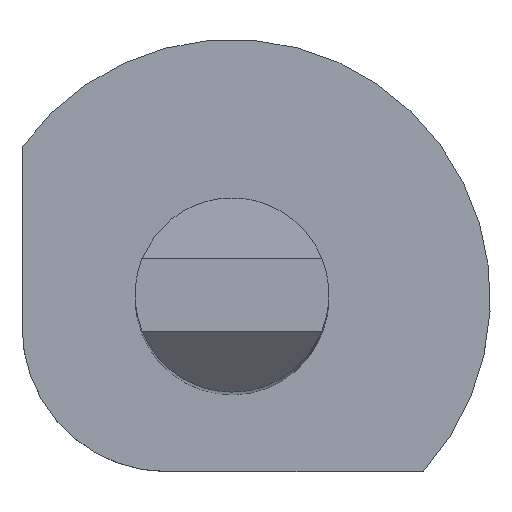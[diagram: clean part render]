
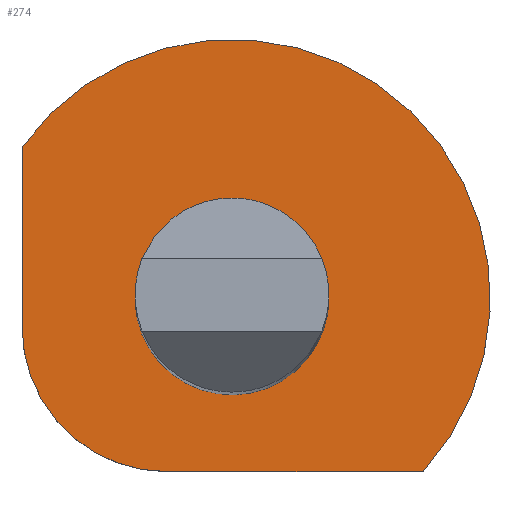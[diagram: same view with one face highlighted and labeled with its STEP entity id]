
A CAD part, top view. The second image highlights one B-rep face of the part: STEP entity #274.
In plain terms, the highlighted planar face has unit normal (0, 0, 1).
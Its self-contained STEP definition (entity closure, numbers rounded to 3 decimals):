
#157=CARTESIAN_POINT('',(2.641,-2.4,0.0));
#158=VERTEX_POINT('',#157);
#165=CARTESIAN_POINT('',(-0.9,-2.4,0.0));
#166=VERTEX_POINT('',#165);
#167=CARTESIAN_POINT('',(2.641,-2.4,0.0));
#168=DIRECTION('',(-1.0,0.0,0.0));
#169=VECTOR('',#168,3.541);
#170=LINE('',#167,#169);
#171=EDGE_CURVE('',#158,#166,#170,.T.);
#197=CARTESIAN_POINT('',(-2.9,-0.4,0.0));
#198=VERTEX_POINT('',#197);
#199=CARTESIAN_POINT('',(-0.9,-0.4,0.0));
#200=DIRECTION('',(0.0,0.0,-1.0));
#201=DIRECTION('',(1.0,0.0,0.0));
#202=AXIS2_PLACEMENT_3D('',#199,#200,#201);
#203=CIRCLE('',#202,2.0);
#204=EDGE_CURVE('',#166,#198,#203,.T.);
#229=CARTESIAN_POINT('',(-2.9,2.08,0.0));
#230=VERTEX_POINT('',#229);
#231=CARTESIAN_POINT('',(-2.9,-0.4,0.0));
#232=DIRECTION('',(0.0,1.0,0.0));
#233=VECTOR('',#232,2.48);
#234=LINE('',#231,#233);
#235=EDGE_CURVE('',#198,#230,#234,.T.);
#246=CARTESIAN_POINT('',(0.0,0.0,0.0));
#247=DIRECTION('',(0.0,0.0,-1.0));
#248=DIRECTION('',(-1.0,0.0,0.0));
#249=AXIS2_PLACEMENT_3D('',#246,#247,#248);
#250=PLANE('',#249);
#251=ORIENTED_EDGE('',*,*,#235,.F.);
#252=ORIENTED_EDGE('',*,*,#204,.F.);
#253=ORIENTED_EDGE('',*,*,#171,.F.);
#254=CARTESIAN_POINT('',(0.0,0.0,0.0));
#255=DIRECTION('',(0.0,0.0,-1.0));
#256=DIRECTION('',(-1.0,0.0,0.0));
#257=AXIS2_PLACEMENT_3D('',#254,#255,#256);
#258=CIRCLE('',#257,3.569);
#259=EDGE_CURVE('',#230,#158,#258,.T.);
#260=ORIENTED_EDGE('',*,*,#259,.F.);
#261=EDGE_LOOP('',(#251,#252,#253,#260));
#262=FACE_OUTER_BOUND('',#261,.T.);
#263=CARTESIAN_POINT('',(1.34,0.,0.0));
#264=VERTEX_POINT('',#263);
#265=CARTESIAN_POINT('',(0.0,0.0,0.0));
#266=DIRECTION('',(0.0,0.0,-1.0));
#267=DIRECTION('',(-1.0,0.0,0.0));
#268=AXIS2_PLACEMENT_3D('',#265,#266,#267);
#269=CIRCLE('',#268,1.34);
#270=EDGE_CURVE('',#264,#264,#269,.T.);
#271=ORIENTED_EDGE('',*,*,#270,.T.);
#272=EDGE_LOOP('',(#271));
#273=FACE_BOUND('',#272,.T.);
#274=ADVANCED_FACE('',(#262,#273),#250,.F.);
